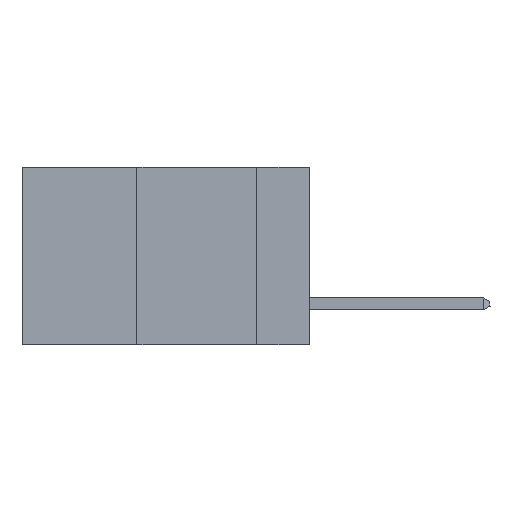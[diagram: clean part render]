
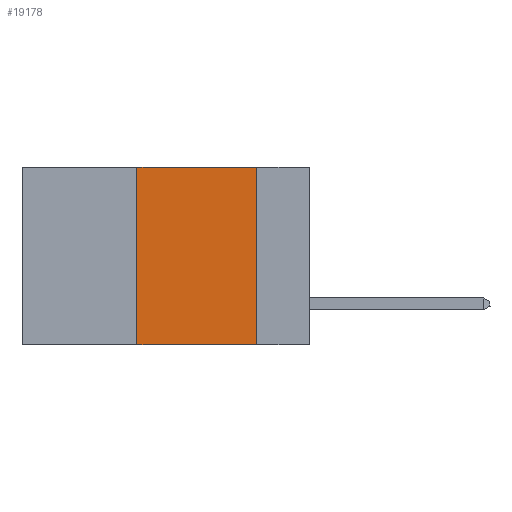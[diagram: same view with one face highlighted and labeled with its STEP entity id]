
A CAD part, left-side view. The second image highlights one B-rep face of the part: STEP entity #19178.
In plain terms, the highlighted planar face has unit normal (-1, 0, 0).
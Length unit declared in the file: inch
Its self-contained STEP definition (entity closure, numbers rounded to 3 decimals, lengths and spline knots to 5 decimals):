
#2360 = EDGE_CURVE ( 'NONE', #20368, #2676, #17720, .T. ) ;
#2598 = AXIS2_PLACEMENT_3D ( 'NONE', #12863, #8390, #10088 ) ;
#2676 = VERTEX_POINT ( 'NONE', #10890 ) ;
#3125 = DIRECTION ( 'NONE',  ( 0., 0., 1. ) ) ;
#3157 = VECTOR ( 'NONE', #3125, 39.37008 ) ;
#3432 = ORIENTED_EDGE ( 'NONE', *, *, #18893, .F. ) ;
#3766 = CARTESIAN_POINT ( 'NONE',  ( 0., 0.11, 0. ) ) ;
#3894 = VECTOR ( 'NONE', #9820, 39.37008 ) ;
#5056 = CARTESIAN_POINT ( 'NONE',  ( 0., 0.36, 0. ) ) ;
#5298 = CARTESIAN_POINT ( 'NONE',  ( 0., 0.36, -0.37 ) ) ;
#6831 = DIRECTION ( 'NONE',  ( 0., -1., 0. ) ) ;
#6869 = CARTESIAN_POINT ( 'NONE',  ( 0., 0.11, -0.37 ) ) ;
#7177 = ORIENTED_EDGE ( 'NONE', *, *, #16918, .F. ) ;
#8390 = DIRECTION ( 'NONE',  ( 1., 0., 0. ) ) ;
#8757 = VERTEX_POINT ( 'NONE', #3766 ) ;
#9820 = DIRECTION ( 'NONE',  ( 0., -1., 0. ) ) ;
#9994 = VERTEX_POINT ( 'NONE', #6869 ) ;
#10088 = DIRECTION ( 'NONE',  ( 0., 0., -1. ) ) ;
#10526 = EDGE_CURVE ( 'NONE', #20368, #9994, #19713, .T. ) ;
#10569 = ORIENTED_EDGE ( 'NONE', *, *, #2360, .F. ) ;
#10890 = CARTESIAN_POINT ( 'NONE',  ( 0., 0.36, 0. ) ) ;
#12863 = CARTESIAN_POINT ( 'NONE',  ( 0., 0.6, 0. ) ) ;
#14368 = LINE ( 'NONE', #16394, #3894 ) ;
#15392 = CARTESIAN_POINT ( 'NONE',  ( 0., 0.11, 0. ) ) ;
#15929 = ORIENTED_EDGE ( 'NONE', *, *, #10526, .T. ) ;
#16148 = FACE_OUTER_BOUND ( 'NONE', #21037, .T. ) ;
#16394 = CARTESIAN_POINT ( 'NONE',  ( 0., 0.6, 0. ) ) ;
#16553 = VECTOR ( 'NONE', #6831, 39.37008 ) ;
#16717 = CARTESIAN_POINT ( 'NONE',  ( 0., 0.6, -0.37 ) ) ;
#16912 = LINE ( 'NONE', #15392, #19631 ) ;
#16918 = EDGE_CURVE ( 'NONE', #2676, #8757, #14368, .T. ) ;
#17720 = LINE ( 'NONE', #5056, #3157 ) ;
#18893 = EDGE_CURVE ( 'NONE', #8757, #9994, #16912, .T. ) ;
#19178 = ADVANCED_FACE ( 'NONE', ( #16148 ), #20951, .F. ) ;
#19631 = VECTOR ( 'NONE', #20201, 39.37008 ) ;
#19713 = LINE ( 'NONE', #16717, #16553 ) ;
#20201 = DIRECTION ( 'NONE',  ( 0., 0., -1. ) ) ;
#20368 = VERTEX_POINT ( 'NONE', #5298 ) ;
#20951 = PLANE ( 'NONE',  #2598 ) ;
#21037 = EDGE_LOOP ( 'NONE', ( #3432, #7177, #10569, #15929 ) ) ;
